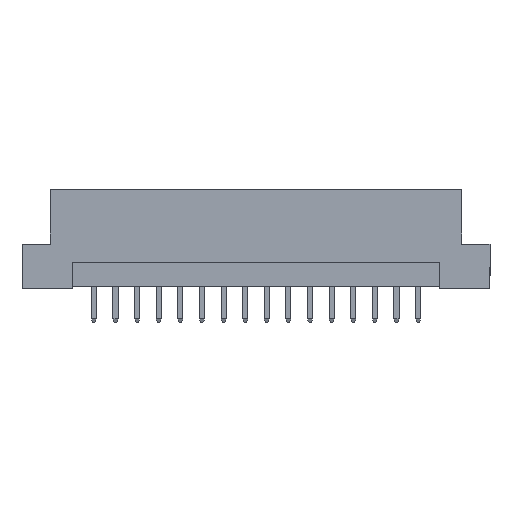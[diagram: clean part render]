
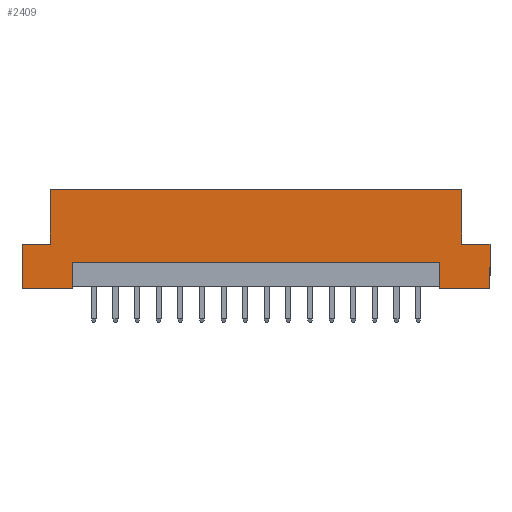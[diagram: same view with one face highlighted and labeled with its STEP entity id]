
A CAD part, front view. The second image highlights one B-rep face of the part: STEP entity #2409.
In plain terms, the highlighted planar face has unit normal (0, -1, 0).
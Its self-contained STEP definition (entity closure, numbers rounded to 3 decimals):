
#70 = VERTEX_POINT ( 'NONE', #798 ) ;
#98 = CARTESIAN_POINT ( 'NONE',  ( -27.5, -4.3, 5.2 ) ) ;
#214 = ORIENTED_EDGE ( 'NONE', *, *, #2957, .F. ) ;
#333 = ORIENTED_EDGE ( 'NONE', *, *, #1114, .T. ) ;
#337 = VERTEX_POINT ( 'NONE', #6397 ) ;
#375 = CARTESIAN_POINT ( 'NONE',  ( 27.5, -4.3, 11.6 ) ) ;
#414 = VERTEX_POINT ( 'NONE', #2611 ) ;
#516 = DIRECTION ( 'NONE',  ( 0., 0., 1. ) ) ;
#522 = ORIENTED_EDGE ( 'NONE', *, *, #6337, .T. ) ;
#531 = LINE ( 'NONE', #1624, #3752 ) ;
#666 = VECTOR ( 'NONE', #5241, 1000. ) ;
#682 = LINE ( 'NONE', #713, #1516 ) ;
#713 = CARTESIAN_POINT ( 'NONE',  ( 27.5, -4.3, 11.6 ) ) ;
#740 = CARTESIAN_POINT ( 'NONE',  ( 21.6, -4.3, 0. ) ) ;
#756 = VECTOR ( 'NONE', #3467, 1000. ) ;
#794 = VECTOR ( 'NONE', #516, 1000. ) ;
#798 = CARTESIAN_POINT ( 'NONE',  ( 27.5, -4.3, 0. ) ) ;
#831 = LINE ( 'NONE', #375, #6914 ) ;
#1021 = ORIENTED_EDGE ( 'NONE', *, *, #3465, .F. ) ;
#1056 = CARTESIAN_POINT ( 'NONE',  ( -21.6, -4.3, 0.2 ) ) ;
#1114 = EDGE_CURVE ( 'NONE', #6841, #414, #2116, .T. ) ;
#1128 = CARTESIAN_POINT ( 'NONE',  ( -21.6, -4.3, 0. ) ) ;
#1158 = LINE ( 'NONE', #4633, #756 ) ;
#1463 = EDGE_CURVE ( 'NONE', #4995, #7365, #3848, .T. ) ;
#1516 = VECTOR ( 'NONE', #6407, 1000. ) ;
#1549 = CARTESIAN_POINT ( 'NONE',  ( 21.6, -4.3, 3. ) ) ;
#1589 = DIRECTION ( 'NONE',  ( 1., 0., 0. ) ) ;
#1624 = CARTESIAN_POINT ( 'NONE',  ( 27.5, -4.3, 5.2 ) ) ;
#1630 = DIRECTION ( 'NONE',  ( 0., 0., -1. ) ) ;
#1716 = EDGE_CURVE ( 'NONE', #5112, #70, #682, .T. ) ;
#2009 = DIRECTION ( 'NONE',  ( 1., 0., 0. ) ) ;
#2116 = LINE ( 'NONE', #6817, #3267 ) ;
#2192 = VECTOR ( 'NONE', #2636, 1000. ) ;
#2213 = CARTESIAN_POINT ( 'NONE',  ( -21.6, -4.3, 3. ) ) ;
#2239 = EDGE_CURVE ( 'NONE', #6841, #3726, #6869, .T. ) ;
#2249 = LINE ( 'NONE', #1056, #3047 ) ;
#2398 = AXIS2_PLACEMENT_3D ( 'NONE', #3676, #7066, #2463 ) ;
#2409 = ADVANCED_FACE ( 'NONE', ( #4426 ), #4745, .F. ) ;
#2425 = CARTESIAN_POINT ( 'NONE',  ( -24.2, -4.3, 5.2 ) ) ;
#2463 = DIRECTION ( 'NONE',  ( -1., 0., 0. ) ) ;
#2567 = CARTESIAN_POINT ( 'NONE',  ( -24.2, -4.3, 5.2 ) ) ;
#2610 = CARTESIAN_POINT ( 'NONE',  ( -21.6, -4.3, 3. ) ) ;
#2611 = CARTESIAN_POINT ( 'NONE',  ( -27.5, -4.3, 0. ) ) ;
#2636 = DIRECTION ( 'NONE',  ( 0., 0., 1. ) ) ;
#2679 = CARTESIAN_POINT ( 'NONE',  ( 27.5, -4.3, 0. ) ) ;
#2718 = DIRECTION ( 'NONE',  ( 0., 0., -1. ) ) ;
#2777 = CARTESIAN_POINT ( 'NONE',  ( 21.6, -4.3, 0.2 ) ) ;
#2790 = EDGE_CURVE ( 'NONE', #4233, #3647, #831, .T. ) ;
#2835 = EDGE_CURVE ( 'NONE', #3726, #4233, #6117, .T. ) ;
#2946 = VERTEX_POINT ( 'NONE', #1128 ) ;
#2957 = EDGE_CURVE ( 'NONE', #4995, #2946, #2249, .T. ) ;
#3017 = ORIENTED_EDGE ( 'NONE', *, *, #5649, .F. ) ;
#3047 = VECTOR ( 'NONE', #2718, 1000. ) ;
#3052 = VECTOR ( 'NONE', #6042, 1000. ) ;
#3267 = VECTOR ( 'NONE', #1630, 1000. ) ;
#3315 = VECTOR ( 'NONE', #6156, 1000. ) ;
#3465 = EDGE_CURVE ( 'NONE', #3886, #7365, #6721, .T. ) ;
#3467 = DIRECTION ( 'NONE',  ( 0., 0., 1. ) ) ;
#3647 = VERTEX_POINT ( 'NONE', #6836 ) ;
#3676 = CARTESIAN_POINT ( 'NONE',  ( 27.5, -4.3, 11.6 ) ) ;
#3726 = VERTEX_POINT ( 'NONE', #2425 ) ;
#3752 = VECTOR ( 'NONE', #1589, 1000. ) ;
#3848 = LINE ( 'NONE', #2213, #3315 ) ;
#3886 = VERTEX_POINT ( 'NONE', #740 ) ;
#4095 = VECTOR ( 'NONE', #2009, 1000. ) ;
#4169 = CARTESIAN_POINT ( 'NONE',  ( -27.5, -4.3, 5.2 ) ) ;
#4229 = DIRECTION ( 'NONE',  ( 1., 0., 0. ) ) ;
#4233 = VERTEX_POINT ( 'NONE', #4553 ) ;
#4426 = FACE_OUTER_BOUND ( 'NONE', #5180, .T. ) ;
#4541 = ORIENTED_EDGE ( 'NONE', *, *, #5018, .T. ) ;
#4553 = CARTESIAN_POINT ( 'NONE',  ( -24.2, -4.3, 11.6 ) ) ;
#4633 = CARTESIAN_POINT ( 'NONE',  ( 24.2, -4.3, 5.2 ) ) ;
#4745 = PLANE ( 'NONE',  #2398 ) ;
#4777 = ORIENTED_EDGE ( 'NONE', *, *, #2790, .F. ) ;
#4898 = LINE ( 'NONE', #7203, #4095 ) ;
#4995 = VERTEX_POINT ( 'NONE', #2610 ) ;
#5018 = EDGE_CURVE ( 'NONE', #3886, #70, #4898, .T. ) ;
#5112 = VERTEX_POINT ( 'NONE', #7394 ) ;
#5180 = EDGE_LOOP ( 'NONE', ( #6531, #1021, #4541, #5592, #3017, #522, #4777, #7406, #6115, #333, #7142, #214 ) ) ;
#5241 = DIRECTION ( 'NONE',  ( 1., 0., 0. ) ) ;
#5592 = ORIENTED_EDGE ( 'NONE', *, *, #1716, .F. ) ;
#5649 = EDGE_CURVE ( 'NONE', #337, #5112, #531, .T. ) ;
#6042 = DIRECTION ( 'NONE',  ( 1., 0., 0. ) ) ;
#6115 = ORIENTED_EDGE ( 'NONE', *, *, #2239, .F. ) ;
#6117 = LINE ( 'NONE', #2567, #2192 ) ;
#6156 = DIRECTION ( 'NONE',  ( 1., 0., 0. ) ) ;
#6337 = EDGE_CURVE ( 'NONE', #337, #3647, #1158, .T. ) ;
#6397 = CARTESIAN_POINT ( 'NONE',  ( 24.2, -4.3, 5.2 ) ) ;
#6407 = DIRECTION ( 'NONE',  ( 0., 0., -1. ) ) ;
#6531 = ORIENTED_EDGE ( 'NONE', *, *, #1463, .T. ) ;
#6695 = LINE ( 'NONE', #2679, #3052 ) ;
#6721 = LINE ( 'NONE', #2777, #794 ) ;
#6817 = CARTESIAN_POINT ( 'NONE',  ( -27.5, -4.3, 11.6 ) ) ;
#6836 = CARTESIAN_POINT ( 'NONE',  ( 24.2, -4.3, 11.6 ) ) ;
#6841 = VERTEX_POINT ( 'NONE', #4169 ) ;
#6869 = LINE ( 'NONE', #98, #666 ) ;
#6914 = VECTOR ( 'NONE', #4229, 1000. ) ;
#6958 = EDGE_CURVE ( 'NONE', #414, #2946, #6695, .T. ) ;
#7066 = DIRECTION ( 'NONE',  ( 0., 1., 0. ) ) ;
#7142 = ORIENTED_EDGE ( 'NONE', *, *, #6958, .T. ) ;
#7203 = CARTESIAN_POINT ( 'NONE',  ( 27.5, -4.3, 0. ) ) ;
#7365 = VERTEX_POINT ( 'NONE', #1549 ) ;
#7394 = CARTESIAN_POINT ( 'NONE',  ( 27.5, -4.3, 5.2 ) ) ;
#7406 = ORIENTED_EDGE ( 'NONE', *, *, #2835, .F. ) ;
